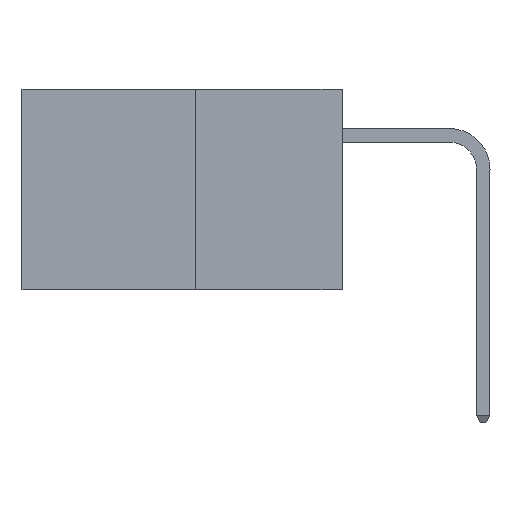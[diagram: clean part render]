
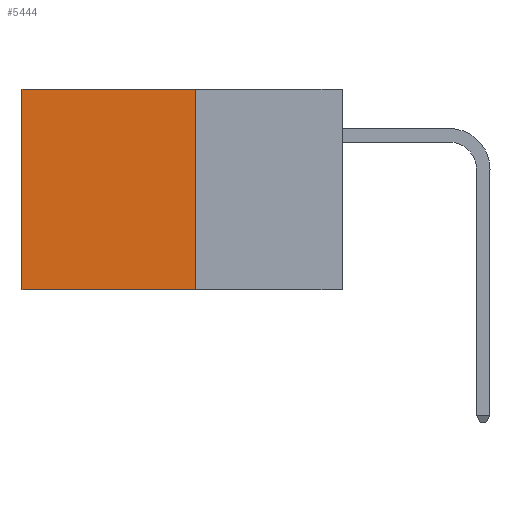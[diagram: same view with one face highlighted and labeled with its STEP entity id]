
A CAD part, left-side view. The second image highlights one B-rep face of the part: STEP entity #5444.
In plain terms, the highlighted planar face has unit normal (-1, 0, 0).
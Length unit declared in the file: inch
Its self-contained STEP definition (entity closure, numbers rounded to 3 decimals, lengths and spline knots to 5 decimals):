
#243 = EDGE_LOOP ( 'NONE', ( #1992, #4716, #12233, #2321 ) ) ;
#534 = VERTEX_POINT ( 'NONE', #7260 ) ;
#1533 = CARTESIAN_POINT ( 'NONE',  ( 0.277, 0.59, -0.37 ) ) ;
#1992 = ORIENTED_EDGE ( 'NONE', *, *, #7610, .T. ) ;
#2321 = ORIENTED_EDGE ( 'NONE', *, *, #2600, .T. ) ;
#2600 = EDGE_CURVE ( 'NONE', #534, #3450, #8530, .T. ) ;
#2732 = DIRECTION ( 'NONE',  ( 0., 0., -1. ) ) ;
#2902 = CARTESIAN_POINT ( 'NONE',  ( 0.277, 0.27, 0. ) ) ;
#2968 = DIRECTION ( 'NONE',  ( 0., 1., 0. ) ) ;
#3275 = FACE_OUTER_BOUND ( 'NONE', #243, .T. ) ;
#3450 = VERTEX_POINT ( 'NONE', #11738 ) ;
#4716 = ORIENTED_EDGE ( 'NONE', *, *, #11424, .F. ) ;
#4752 = CARTESIAN_POINT ( 'NONE',  ( 0.277, 0.27, -0.37 ) ) ;
#5444 = ADVANCED_FACE ( 'NONE', ( #3275 ), #11571, .F. ) ;
#5586 = LINE ( 'NONE', #7390, #10323 ) ;
#5790 = AXIS2_PLACEMENT_3D ( 'NONE', #11556, #11532, #11449 ) ;
#6459 = LINE ( 'NONE', #11299, #11114 ) ;
#6716 = DIRECTION ( 'NONE',  ( 0., 1., 0. ) ) ;
#7260 = CARTESIAN_POINT ( 'NONE',  ( 0.277, 0.27, 0. ) ) ;
#7358 = LINE ( 'NONE', #4752, #9226 ) ;
#7390 = CARTESIAN_POINT ( 'NONE',  ( 0.277, 0.59, -0.37 ) ) ;
#7610 = EDGE_CURVE ( 'NONE', #3450, #11430, #5586, .T. ) ;
#7954 = EDGE_CURVE ( 'NONE', #534, #11911, #7358, .T. ) ;
#8348 = DIRECTION ( 'NONE',  ( 0., 0., -1. ) ) ;
#8530 = LINE ( 'NONE', #2902, #10645 ) ;
#9226 = VECTOR ( 'NONE', #2732, 39.37008 ) ;
#10059 = CARTESIAN_POINT ( 'NONE',  ( 0.277, 0.27, -0.37 ) ) ;
#10323 = VECTOR ( 'NONE', #8348, 39.37008 ) ;
#10645 = VECTOR ( 'NONE', #2968, 39.37008 ) ;
#11114 = VECTOR ( 'NONE', #6716, 39.37008 ) ;
#11299 = CARTESIAN_POINT ( 'NONE',  ( 0.277, 0.27, -0.37 ) ) ;
#11424 = EDGE_CURVE ( 'NONE', #11911, #11430, #6459, .T. ) ;
#11430 = VERTEX_POINT ( 'NONE', #1533 ) ;
#11449 = DIRECTION ( 'NONE',  ( 0., 0., -1. ) ) ;
#11532 = DIRECTION ( 'NONE',  ( 1., 0., 0. ) ) ;
#11556 = CARTESIAN_POINT ( 'NONE',  ( 0.277, 0.27, -0.37 ) ) ;
#11571 = PLANE ( 'NONE',  #5790 ) ;
#11738 = CARTESIAN_POINT ( 'NONE',  ( 0.277, 0.59, 0. ) ) ;
#11911 = VERTEX_POINT ( 'NONE', #10059 ) ;
#12233 = ORIENTED_EDGE ( 'NONE', *, *, #7954, .F. ) ;
